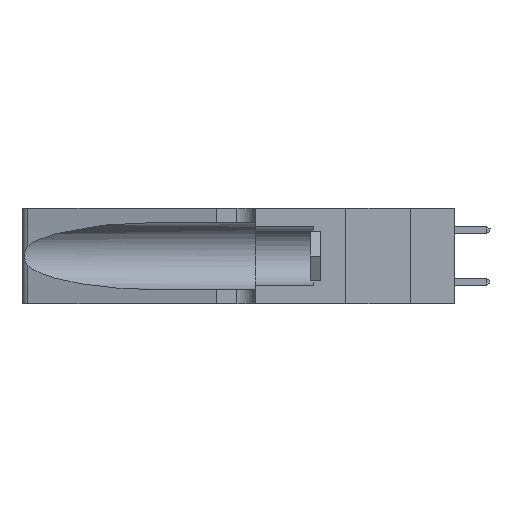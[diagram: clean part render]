
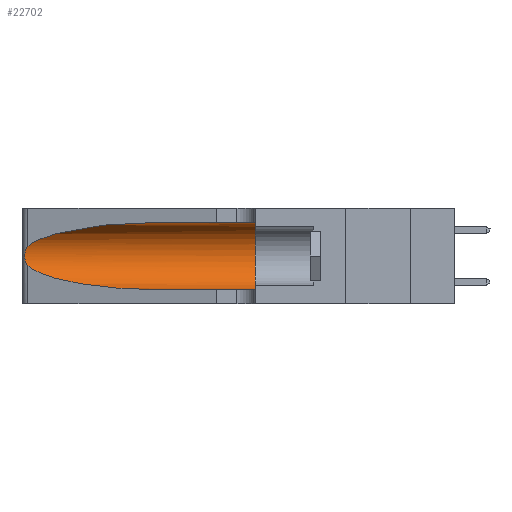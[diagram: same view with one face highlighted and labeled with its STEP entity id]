
A CAD part, left-side view. The second image highlights one B-rep face of the part: STEP entity #22702.
In plain terms, the highlighted cylindrical face has radius 3.308 mm (diameter 6.617 mm), a partial arc.
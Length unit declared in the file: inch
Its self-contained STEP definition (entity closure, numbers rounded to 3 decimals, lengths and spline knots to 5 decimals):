
#29 = EDGE_CURVE ( 'NONE', #754, #8375, #22358, .T. ) ;
#165 = CARTESIAN_POINT ( 'NONE',  ( 0.1305, 0.72297, 0.31525 ) ) ;
#754 = VERTEX_POINT ( 'NONE', #11321 ) ;
#1018 = EDGE_CURVE ( 'NONE', #9372, #7177, #13056, .T. ) ;
#1131 = ORIENTED_EDGE ( 'NONE', *, *, #25342, .T. ) ;
#1224 = VECTOR ( 'NONE', #1902, 39.37008 ) ;
#1472 = CARTESIAN_POINT ( 'NONE',  ( 0.25487, 1.22718, 0.14631 ) ) ;
#1902 = DIRECTION ( 'NONE',  ( 0., -1., 0. ) ) ;
#2821 = CARTESIAN_POINT ( 'NONE',  ( 0.1305, 1.61858, 0.05475 ) ) ;
#3827 = CARTESIAN_POINT ( 'NONE',  ( 0.26075, 1.23896, 0.19203 ) ) ;
#4083 = CARTESIAN_POINT ( 'NONE',  ( 0.2373, 1.15595, 0.28018 ) ) ;
#4240 = AXIS2_PLACEMENT_3D ( 'NONE', #12128, #24412, #16075 ) ;
#4582 = DIRECTION ( 'NONE',  ( 0., 1., 0. ) ) ;
#5002 = VERTEX_POINT ( 'NONE', #19029 ) ;
#5571 = CARTESIAN_POINT ( 'NONE',  ( 0.25555, 1.22993, 0.14849 ) ) ;
#5662 = CARTESIAN_POINT ( 'NONE',  ( 0.26018, 1.23835, 0.19895 ) ) ;
#5937 = CARTESIAN_POINT ( 'NONE',  ( 0.25487, 1.22718, 0.22369 ) ) ;
#6195 = EDGE_CURVE ( 'NONE', #7177, #22388, #25956, .T. ) ;
#7019 = CARTESIAN_POINT ( 'NONE',  ( 0.1305, 0.72297, 0.05475 ) ) ;
#7177 = VERTEX_POINT ( 'NONE', #22132 ) ;
#7626 = CARTESIAN_POINT ( 'NONE',  ( 0.25487, 1.22718, 0.22369 ) ) ;
#7661 = EDGE_CURVE ( 'NONE', #8375, #5002, #14865, .T. ) ;
#7669 = ORIENTED_EDGE ( 'NONE', *, *, #1018, .F. ) ;
#7718 = CARTESIAN_POINT ( 'NONE',  ( 0.25789, 1.23486, 0.15765 ) ) ;
#7917 = CARTESIAN_POINT ( 'NONE',  ( 0.1305, 1.61858, 0.31525 ) ) ;
#8375 = VERTEX_POINT ( 'NONE', #1472 ) ;
#8596 =( BOUNDED_CURVE ( )  B_SPLINE_CURVE ( 3, ( #23885, #26009, #4083, #5937 ),
 .UNSPECIFIED., .F., .F. ) 
 B_SPLINE_CURVE_WITH_KNOTS ( ( 4, 4 ),
 ( 1.5708, 2.84003 ),
 .UNSPECIFIED. ) 
 CURVE ( )  GEOMETRIC_REPRESENTATION_ITEM ( )  RATIONAL_B_SPLINE_CURVE ( ( 1., 0.87, 0.87, 1. ) ) 
 REPRESENTATION_ITEM ( '' )  );
#9372 = VERTEX_POINT ( 'NONE', #165 ) ;
#9623 = EDGE_CURVE ( 'NONE', #5002, #22388, #21350, .T. ) ;
#9649 = CARTESIAN_POINT ( 'NONE',  ( 0.25856, 1.23593, 0.16098 ) ) ;
#10753 = DIRECTION ( 'NONE',  ( 0., -1., 0. ) ) ;
#11321 = CARTESIAN_POINT ( 'NONE',  ( 0.25487, 1.22718, 0.22369 ) ) ;
#11423 = ORIENTED_EDGE ( 'NONE', *, *, #9623, .T. ) ;
#11527 = CARTESIAN_POINT ( 'NONE',  ( 0.2373, 1.15595, 0.08982 ) ) ;
#12128 = CARTESIAN_POINT ( 'NONE',  ( 0.1305, 1.61858, 0.185 ) ) ;
#13056 = LINE ( 'NONE', #7917, #1224 ) ;
#13443 = CARTESIAN_POINT ( 'NONE',  ( 0.1305, 0.35, 0.05475 ) ) ;
#13468 = ORIENTED_EDGE ( 'NONE', *, *, #29, .T. ) ;
#14865 =( BOUNDED_CURVE ( )  B_SPLINE_CURVE ( 3, ( #19868, #11527, #17630, #7019 ),
 .UNSPECIFIED., .F., .T. ) 
 B_SPLINE_CURVE_WITH_KNOTS ( ( 4, 4 ),
 ( 3.44316, 4.71239 ),
 .UNSPECIFIED. ) 
 CURVE ( )  GEOMETRIC_REPRESENTATION_ITEM ( )  RATIONAL_B_SPLINE_CURVE ( ( 1., 0.87, 0.87, 1. ) ) 
 REPRESENTATION_ITEM ( '' )  );
#15637 = CARTESIAN_POINT ( 'NONE',  ( 0.26075, 1.23896, 0.178 ) ) ;
#15723 = CARTESIAN_POINT ( 'NONE',  ( 0.26017, 1.23833, 0.17102 ) ) ;
#16075 = DIRECTION ( 'NONE',  ( 0., 0., -1. ) ) ;
#16343 = FACE_OUTER_BOUND ( 'NONE', #16354, .T. ) ;
#16354 = EDGE_LOOP ( 'NONE', ( #1131, #13468, #20481, #11423, #23771, #7669 ) ) ;
#16665 = CARTESIAN_POINT ( 'NONE',  ( 0.1305, 0.35, 0.185 ) ) ;
#16878 = VECTOR ( 'NONE', #10753, 39.37008 ) ;
#17630 = CARTESIAN_POINT ( 'NONE',  ( 0.18966, 0.96281, 0.05475 ) ) ;
#17874 = CARTESIAN_POINT ( 'NONE',  ( 0.25555, 1.22994, 0.2215 ) ) ;
#18730 = DIRECTION ( 'NONE',  ( 0., 0., 1. ) ) ;
#19029 = CARTESIAN_POINT ( 'NONE',  ( 0.1305, 0.72297, 0.05475 ) ) ;
#19265 = CYLINDRICAL_SURFACE ( 'NONE', #4240, 0.13025 ) ;
#19658 = CARTESIAN_POINT ( 'NONE',  ( 0.25639, 1.23184, 0.21858 ) ) ;
#19868 = CARTESIAN_POINT ( 'NONE',  ( 0.25487, 1.22718, 0.14631 ) ) ;
#19926 = CARTESIAN_POINT ( 'NONE',  ( 0.25787, 1.23484, 0.2124 ) ) ;
#20481 = ORIENTED_EDGE ( 'NONE', *, *, #7661, .T. ) ;
#21350 = LINE ( 'NONE', #2821, #16878 ) ;
#22132 = CARTESIAN_POINT ( 'NONE',  ( 0.1305, 0.35, 0.31525 ) ) ;
#22358 = B_SPLINE_CURVE_WITH_KNOTS ( 'NONE', 3,
 ( #7626, #17874, #19658, #19926, #26012, #5662, #3827, #15637, #15723, #9649, #7718, #23797, #5571, #25746 ),
 .UNSPECIFIED., .F., .F.,
 ( 4, 2, 2, 2, 2, 2, 4 ),
 ( 0., 0.00027, 0.00053, 0.00107, 0.0016, 0.00187, 0.00214 ),
 .UNSPECIFIED. ) ;
#22388 = VERTEX_POINT ( 'NONE', #13443 ) ;
#22702 = ADVANCED_FACE ( 'NONE', ( #16343 ), #19265, .F. ) ;
#23771 = ORIENTED_EDGE ( 'NONE', *, *, #6195, .F. ) ;
#23797 = CARTESIAN_POINT ( 'NONE',  ( 0.25639, 1.23186, 0.15144 ) ) ;
#23885 = CARTESIAN_POINT ( 'NONE',  ( 0.1305, 0.72297, 0.31525 ) ) ;
#23913 = AXIS2_PLACEMENT_3D ( 'NONE', #16665, #4582, #18730 ) ;
#24412 = DIRECTION ( 'NONE',  ( 0., -1., 0. ) ) ;
#25342 = EDGE_CURVE ( 'NONE', #9372, #754, #8596, .T. ) ;
#25746 = CARTESIAN_POINT ( 'NONE',  ( 0.25487, 1.22718, 0.14631 ) ) ;
#25956 = CIRCLE ( 'NONE', #23913, 0.13025 ) ;
#26009 = CARTESIAN_POINT ( 'NONE',  ( 0.18966, 0.96281, 0.31525 ) ) ;
#26012 = CARTESIAN_POINT ( 'NONE',  ( 0.25854, 1.2359, 0.20912 ) ) ;
